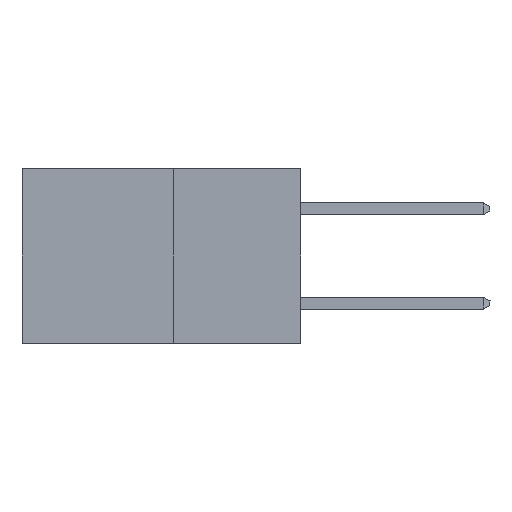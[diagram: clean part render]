
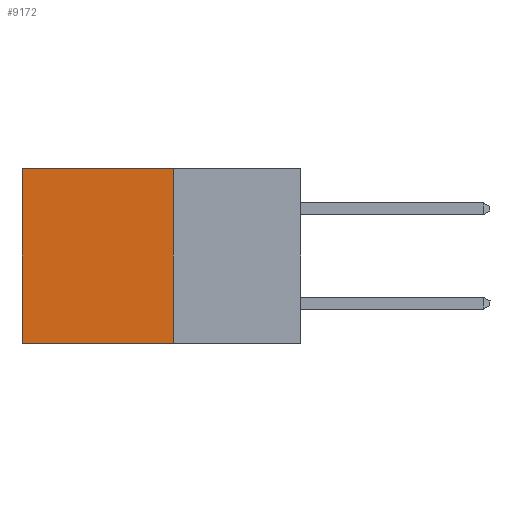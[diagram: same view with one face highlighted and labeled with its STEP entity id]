
A CAD part, left-side view. The second image highlights one B-rep face of the part: STEP entity #9172.
In plain terms, the highlighted planar face has unit normal (-1, 0, 0).
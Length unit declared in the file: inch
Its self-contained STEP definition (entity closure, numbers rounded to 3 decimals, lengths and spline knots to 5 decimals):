
#34 = VECTOR ( 'NONE', #3732, 39.37008 ) ;
#131 = VERTEX_POINT ( 'NONE', #3830 ) ;
#219 = FACE_OUTER_BOUND ( 'NONE', #8948, .T. ) ;
#249 = DIRECTION ( 'NONE',  ( 0., 0., -1. ) ) ;
#301 = VERTEX_POINT ( 'NONE', #9340 ) ;
#1328 = DIRECTION ( 'NONE',  ( 0., 0., -1. ) ) ;
#1694 = ORIENTED_EDGE ( 'NONE', *, *, #3884, .F. ) ;
#1959 = CARTESIAN_POINT ( 'NONE',  ( 0.277, 0.59, -0.37 ) ) ;
#2316 = VERTEX_POINT ( 'NONE', #8063 ) ;
#2582 = LINE ( 'NONE', #2863, #4261 ) ;
#2863 = CARTESIAN_POINT ( 'NONE',  ( 0.277, 0.27, 0. ) ) ;
#3259 = CARTESIAN_POINT ( 'NONE',  ( 0.277, 0.27, -0.37 ) ) ;
#3732 = DIRECTION ( 'NONE',  ( 0., 1., 0. ) ) ;
#3830 = CARTESIAN_POINT ( 'NONE',  ( 0.277, 0.59, 0. ) ) ;
#3884 = EDGE_CURVE ( 'NONE', #301, #2316, #6040, .T. ) ;
#4128 = PLANE ( 'NONE',  #9038 ) ;
#4159 = VECTOR ( 'NONE', #1328, 39.37008 ) ;
#4261 = VECTOR ( 'NONE', #9153, 39.37008 ) ;
#4853 = DIRECTION ( 'NONE',  ( 1., 0., 0. ) ) ;
#5047 = VERTEX_POINT ( 'NONE', #6212 ) ;
#5158 = ORIENTED_EDGE ( 'NONE', *, *, #7577, .T. ) ;
#6012 = LINE ( 'NONE', #1959, #4159 ) ;
#6040 = LINE ( 'NONE', #3259, #34 ) ;
#6212 = CARTESIAN_POINT ( 'NONE',  ( 0.277, 0.27, 0. ) ) ;
#6671 = VECTOR ( 'NONE', #6712, 39.37008 ) ;
#6712 = DIRECTION ( 'NONE',  ( 0., 0., -1. ) ) ;
#6933 = ORIENTED_EDGE ( 'NONE', *, *, #7337, .T. ) ;
#7337 = EDGE_CURVE ( 'NONE', #131, #2316, #6012, .T. ) ;
#7577 = EDGE_CURVE ( 'NONE', #5047, #131, #2582, .T. ) ;
#8063 = CARTESIAN_POINT ( 'NONE',  ( 0.277, 0.59, -0.37 ) ) ;
#8338 = CARTESIAN_POINT ( 'NONE',  ( 0.277, 0.27, -0.37 ) ) ;
#8522 = LINE ( 'NONE', #8774, #6671 ) ;
#8643 = ORIENTED_EDGE ( 'NONE', *, *, #8661, .F. ) ;
#8661 = EDGE_CURVE ( 'NONE', #5047, #301, #8522, .T. ) ;
#8774 = CARTESIAN_POINT ( 'NONE',  ( 0.277, 0.27, -0.37 ) ) ;
#8948 = EDGE_LOOP ( 'NONE', ( #6933, #1694, #8643, #5158 ) ) ;
#9038 = AXIS2_PLACEMENT_3D ( 'NONE', #8338, #4853, #249 ) ;
#9153 = DIRECTION ( 'NONE',  ( 0., 1., 0. ) ) ;
#9172 = ADVANCED_FACE ( 'NONE', ( #219 ), #4128, .F. ) ;
#9340 = CARTESIAN_POINT ( 'NONE',  ( 0.277, 0.27, -0.37 ) ) ;
